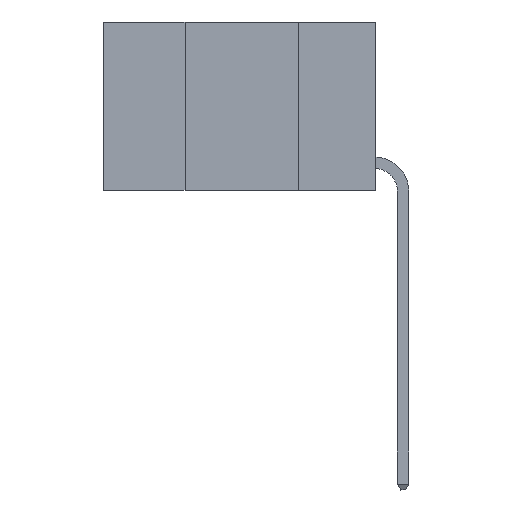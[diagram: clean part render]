
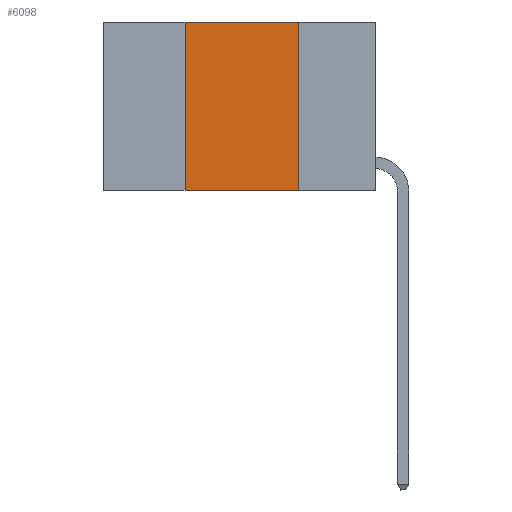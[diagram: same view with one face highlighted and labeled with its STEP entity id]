
A CAD part, left-side view. The second image highlights one B-rep face of the part: STEP entity #6098.
In plain terms, the highlighted planar face has unit normal (-1, 0, 0).
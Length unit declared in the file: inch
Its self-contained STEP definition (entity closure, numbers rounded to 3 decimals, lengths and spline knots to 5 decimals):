
#348 = CARTESIAN_POINT ( 'NONE',  ( 0., 0.17, 0. ) ) ;
#362 = VECTOR ( 'NONE', #7320, 39.37008 ) ;
#607 = VERTEX_POINT ( 'NONE', #5524 ) ;
#1287 = ORIENTED_EDGE ( 'NONE', *, *, #3653, .F. ) ;
#1295 = EDGE_CURVE ( 'NONE', #607, #3493, #8940, .T. ) ;
#1320 = DIRECTION ( 'NONE',  ( 1., 0., 0. ) ) ;
#1672 = EDGE_CURVE ( 'NONE', #3493, #6903, #11607, .T. ) ;
#2043 = DIRECTION ( 'NONE',  ( 0., -1., 0. ) ) ;
#2400 = CARTESIAN_POINT ( 'NONE',  ( 0., 0.6, -0.37 ) ) ;
#2641 = ORIENTED_EDGE ( 'NONE', *, *, #1672, .F. ) ;
#2721 = CARTESIAN_POINT ( 'NONE',  ( 0., 0.17, -0.37 ) ) ;
#3260 = VECTOR ( 'NONE', #2043, 39.37008 ) ;
#3493 = VERTEX_POINT ( 'NONE', #348 ) ;
#3653 = EDGE_CURVE ( 'NONE', #7289, #607, #8871, .T. ) ;
#4322 = VECTOR ( 'NONE', #4601, 39.37008 ) ;
#4392 = ORIENTED_EDGE ( 'NONE', *, *, #11784, .T. ) ;
#4601 = DIRECTION ( 'NONE',  ( 0., -1., 0. ) ) ;
#5194 = CARTESIAN_POINT ( 'NONE',  ( 0., 0.6, 0. ) ) ;
#5524 = CARTESIAN_POINT ( 'NONE',  ( 0., 0.42, 0. ) ) ;
#5542 = CARTESIAN_POINT ( 'NONE',  ( 0., 0.42, -0.37 ) ) ;
#5662 = CARTESIAN_POINT ( 'NONE',  ( 0., 0.6, 0. ) ) ;
#5820 = EDGE_LOOP ( 'NONE', ( #2641, #9389, #1287, #4392 ) ) ;
#6098 = ADVANCED_FACE ( 'NONE', ( #8118 ), #7810, .F. ) ;
#6903 = VERTEX_POINT ( 'NONE', #2721 ) ;
#7164 = CARTESIAN_POINT ( 'NONE',  ( 0., 0.42, 0. ) ) ;
#7289 = VERTEX_POINT ( 'NONE', #5542 ) ;
#7320 = DIRECTION ( 'NONE',  ( 0., 0., -1. ) ) ;
#7810 = PLANE ( 'NONE',  #13186 ) ;
#8118 = FACE_OUTER_BOUND ( 'NONE', #5820, .T. ) ;
#8213 = DIRECTION ( 'NONE',  ( 0., 0., 1. ) ) ;
#8697 = CARTESIAN_POINT ( 'NONE',  ( 0., 0.17, 0. ) ) ;
#8837 = DIRECTION ( 'NONE',  ( 0., 0., -1. ) ) ;
#8871 = LINE ( 'NONE', #7164, #10917 ) ;
#8940 = LINE ( 'NONE', #5194, #3260 ) ;
#9389 = ORIENTED_EDGE ( 'NONE', *, *, #1295, .F. ) ;
#9923 = LINE ( 'NONE', #2400, #4322 ) ;
#10917 = VECTOR ( 'NONE', #8213, 39.37008 ) ;
#11607 = LINE ( 'NONE', #8697, #362 ) ;
#11784 = EDGE_CURVE ( 'NONE', #7289, #6903, #9923, .T. ) ;
#13186 = AXIS2_PLACEMENT_3D ( 'NONE', #5662, #1320, #8837 ) ;
